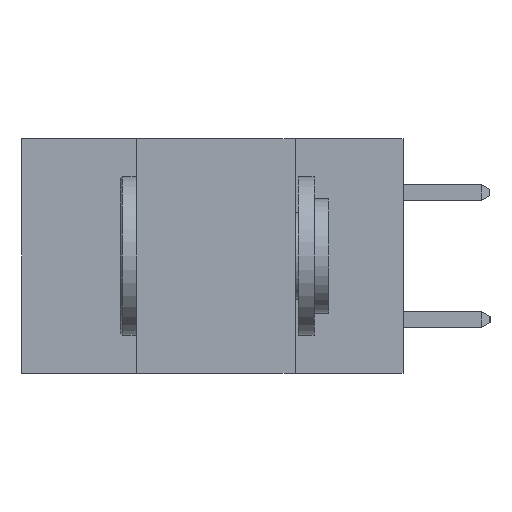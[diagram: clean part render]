
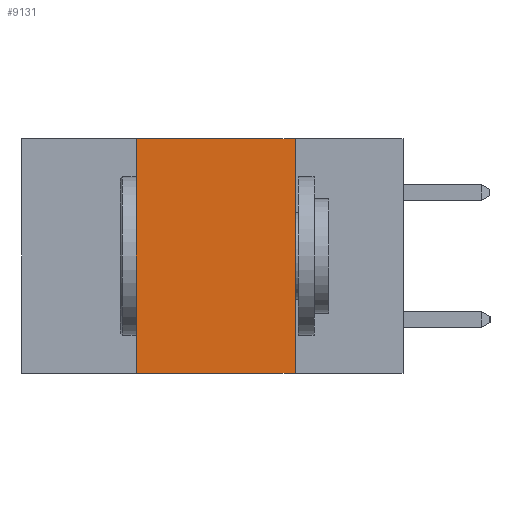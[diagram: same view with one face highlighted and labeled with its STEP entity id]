
A CAD part, left-side view. The second image highlights one B-rep face of the part: STEP entity #9131.
In plain terms, the highlighted planar face has unit normal (-1, 0, 0).
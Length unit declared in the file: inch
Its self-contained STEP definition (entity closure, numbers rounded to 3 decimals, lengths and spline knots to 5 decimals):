
#127 = ORIENTED_EDGE ( 'NONE', *, *, #639, .F. ) ;
#639 = EDGE_CURVE ( 'NONE', #7590, #4784, #2534, .T. ) ;
#776 = DIRECTION ( 'NONE',  ( 0., -1., 0. ) ) ;
#2393 = CARTESIAN_POINT ( 'NONE',  ( 0., 0.17, 0. ) ) ;
#2532 = VECTOR ( 'NONE', #3183, 39.37008 ) ;
#2534 = LINE ( 'NONE', #12962, #6523 ) ;
#3183 = DIRECTION ( 'NONE',  ( 0., -1., 0. ) ) ;
#3228 = FACE_OUTER_BOUND ( 'NONE', #10792, .T. ) ;
#3230 = CARTESIAN_POINT ( 'NONE',  ( 0., 0.6, 0. ) ) ;
#3511 = DIRECTION ( 'NONE',  ( 0., 0., -1. ) ) ;
#3722 = CARTESIAN_POINT ( 'NONE',  ( 0., 0.17, 0. ) ) ;
#4663 = EDGE_CURVE ( 'NONE', #7590, #13017, #12677, .T. ) ;
#4769 = VECTOR ( 'NONE', #776, 39.37008 ) ;
#4784 = VERTEX_POINT ( 'NONE', #5647 ) ;
#4948 = CARTESIAN_POINT ( 'NONE',  ( 0., 0.6, 0. ) ) ;
#5647 = CARTESIAN_POINT ( 'NONE',  ( 0., 0.42, 0. ) ) ;
#6096 = DIRECTION ( 'NONE',  ( 1., 0., 0. ) ) ;
#6523 = VECTOR ( 'NONE', #7485, 39.37008 ) ;
#7064 = PLANE ( 'NONE',  #7306 ) ;
#7116 = EDGE_CURVE ( 'NONE', #11786, #13017, #10745, .T. ) ;
#7126 = ORIENTED_EDGE ( 'NONE', *, *, #4663, .T. ) ;
#7306 = AXIS2_PLACEMENT_3D ( 'NONE', #4948, #6096, #12506 ) ;
#7485 = DIRECTION ( 'NONE',  ( 0., 0., 1. ) ) ;
#7590 = VERTEX_POINT ( 'NONE', #10231 ) ;
#9131 = ADVANCED_FACE ( 'NONE', ( #3228 ), #7064, .F. ) ;
#9187 = EDGE_CURVE ( 'NONE', #4784, #11786, #10132, .T. ) ;
#10132 = LINE ( 'NONE', #3230, #2532 ) ;
#10231 = CARTESIAN_POINT ( 'NONE',  ( 0., 0.42, -0.37 ) ) ;
#10355 = CARTESIAN_POINT ( 'NONE',  ( 0., 0.6, -0.37 ) ) ;
#10745 = LINE ( 'NONE', #2393, #13489 ) ;
#10792 = EDGE_LOOP ( 'NONE', ( #11675, #14025, #127, #7126 ) ) ;
#11675 = ORIENTED_EDGE ( 'NONE', *, *, #7116, .F. ) ;
#11786 = VERTEX_POINT ( 'NONE', #3722 ) ;
#12506 = DIRECTION ( 'NONE',  ( 0., 0., -1. ) ) ;
#12664 = CARTESIAN_POINT ( 'NONE',  ( 0., 0.17, -0.37 ) ) ;
#12677 = LINE ( 'NONE', #10355, #4769 ) ;
#12962 = CARTESIAN_POINT ( 'NONE',  ( 0., 0.42, 0. ) ) ;
#13017 = VERTEX_POINT ( 'NONE', #12664 ) ;
#13489 = VECTOR ( 'NONE', #3511, 39.37008 ) ;
#14025 = ORIENTED_EDGE ( 'NONE', *, *, #9187, .F. ) ;
